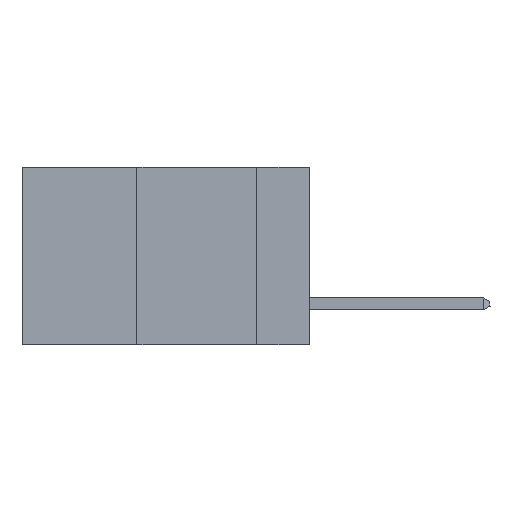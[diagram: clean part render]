
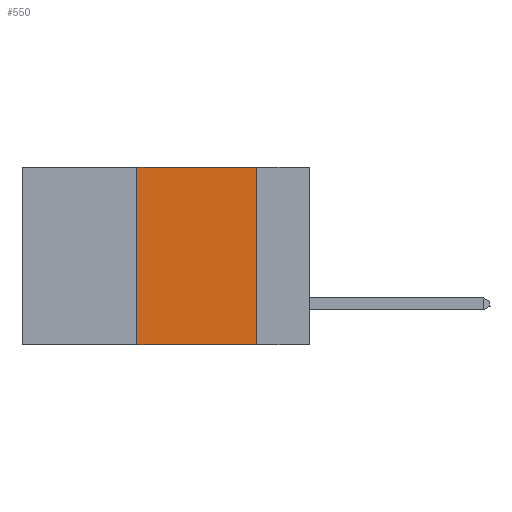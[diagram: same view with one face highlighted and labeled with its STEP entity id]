
A CAD part, left-side view. The second image highlights one B-rep face of the part: STEP entity #550.
In plain terms, the highlighted planar face has unit normal (-1, 0, 0).
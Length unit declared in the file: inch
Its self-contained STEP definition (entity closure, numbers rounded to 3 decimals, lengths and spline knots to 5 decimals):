
#550 = ADVANCED_FACE ( 'NONE', ( #13926 ), #31227, .F. ) ;
#1226 = CARTESIAN_POINT ( 'NONE',  ( 0., 0.11, 0. ) ) ;
#1366 = VECTOR ( 'NONE', #37749, 39.37008 ) ;
#2320 = CARTESIAN_POINT ( 'NONE',  ( 0., 0.11, 0. ) ) ;
#3412 = ORIENTED_EDGE ( 'NONE', *, *, #4586, .F. ) ;
#4586 = EDGE_CURVE ( 'NONE', #4640, #26467, #36816, .T. ) ;
#4640 = VERTEX_POINT ( 'NONE', #18070 ) ;
#6811 = ORIENTED_EDGE ( 'NONE', *, *, #27907, .T. ) ;
#8287 = AXIS2_PLACEMENT_3D ( 'NONE', #21005, #41598, #35119 ) ;
#9214 = CARTESIAN_POINT ( 'NONE',  ( 0., 0.6, -0.37 ) ) ;
#12647 = VECTOR ( 'NONE', #26624, 39.37008 ) ;
#13926 = FACE_OUTER_BOUND ( 'NONE', #36484, .T. ) ;
#15318 = LINE ( 'NONE', #9214, #12647 ) ;
#18070 = CARTESIAN_POINT ( 'NONE',  ( 0., 0.36, 0. ) ) ;
#18603 = DIRECTION ( 'NONE',  ( 0., -1., 0. ) ) ;
#19326 = CARTESIAN_POINT ( 'NONE',  ( 0., 0.36, -0.37 ) ) ;
#21005 = CARTESIAN_POINT ( 'NONE',  ( 0., 0.6, 0. ) ) ;
#21466 = CARTESIAN_POINT ( 'NONE',  ( 0., 0.6, 0. ) ) ;
#21776 = DIRECTION ( 'NONE',  ( 0., 0., -1. ) ) ;
#24517 = VERTEX_POINT ( 'NONE', #35802 ) ;
#26467 = VERTEX_POINT ( 'NONE', #2320 ) ;
#26624 = DIRECTION ( 'NONE',  ( 0., -1., 0. ) ) ;
#27769 = LINE ( 'NONE', #1226, #37998 ) ;
#27816 = CARTESIAN_POINT ( 'NONE',  ( 0., 0.36, 0. ) ) ;
#27839 = EDGE_CURVE ( 'NONE', #26467, #24517, #27769, .T. ) ;
#27907 = EDGE_CURVE ( 'NONE', #44537, #24517, #15318, .T. ) ;
#28737 = VECTOR ( 'NONE', #18603, 39.37008 ) ;
#29871 = EDGE_CURVE ( 'NONE', #44537, #4640, #39208, .T. ) ;
#31227 = PLANE ( 'NONE',  #8287 ) ;
#35119 = DIRECTION ( 'NONE',  ( 0., 0., -1. ) ) ;
#35802 = CARTESIAN_POINT ( 'NONE',  ( 0., 0.11, -0.37 ) ) ;
#36484 = EDGE_LOOP ( 'NONE', ( #44222, #3412, #38069, #6811 ) ) ;
#36816 = LINE ( 'NONE', #21466, #28737 ) ;
#37749 = DIRECTION ( 'NONE',  ( 0., 0., 1. ) ) ;
#37998 = VECTOR ( 'NONE', #21776, 39.37008 ) ;
#38069 = ORIENTED_EDGE ( 'NONE', *, *, #29871, .F. ) ;
#39208 = LINE ( 'NONE', #27816, #1366 ) ;
#41598 = DIRECTION ( 'NONE',  ( 1., 0., 0. ) ) ;
#44222 = ORIENTED_EDGE ( 'NONE', *, *, #27839, .F. ) ;
#44537 = VERTEX_POINT ( 'NONE', #19326 ) ;
